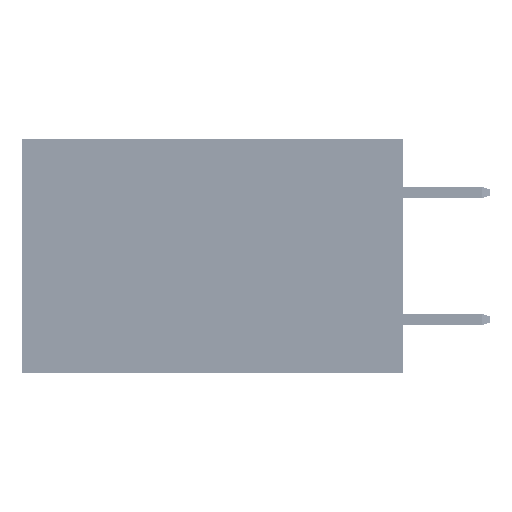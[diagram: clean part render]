
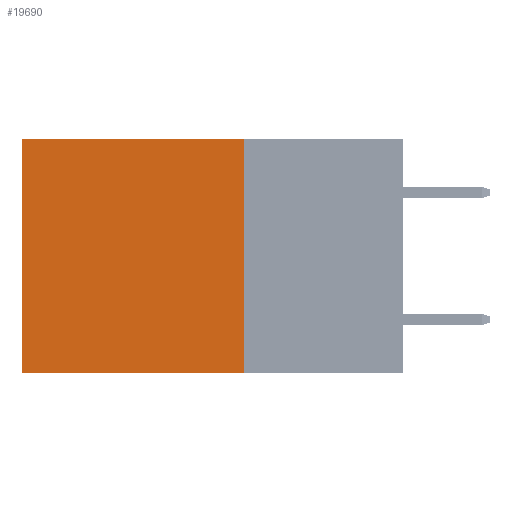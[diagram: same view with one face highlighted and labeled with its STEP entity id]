
A CAD part, left-side view. The second image highlights one B-rep face of the part: STEP entity #19690.
In plain terms, the highlighted planar face has unit normal (-1, 0, 0).
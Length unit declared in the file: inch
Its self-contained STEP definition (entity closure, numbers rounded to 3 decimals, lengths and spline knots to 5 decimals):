
#430 = VECTOR ( 'NONE', #42899, 39.37008 ) ;
#1783 = CARTESIAN_POINT ( 'NONE',  ( 0.2875, 0.6, 0. ) ) ;
#1838 = VECTOR ( 'NONE', #19634, 39.37008 ) ;
#3944 = CARTESIAN_POINT ( 'NONE',  ( 0.2875, 0.25, -0.37 ) ) ;
#4185 = DIRECTION ( 'NONE',  ( 0., 0., -1. ) ) ;
#6712 = DIRECTION ( 'NONE',  ( 0., 0., -1. ) ) ;
#7212 = CARTESIAN_POINT ( 'NONE',  ( 0.2875, 0.25, 0. ) ) ;
#9353 = EDGE_CURVE ( 'NONE', #19038, #37583, #23503, .T. ) ;
#11461 = DIRECTION ( 'NONE',  ( 1., 0., 0. ) ) ;
#12216 = EDGE_CURVE ( 'NONE', #24993, #31007, #19320, .T. ) ;
#14559 = ORIENTED_EDGE ( 'NONE', *, *, #12216, .F. ) ;
#17814 = ORIENTED_EDGE ( 'NONE', *, *, #51083, .F. ) ;
#19038 = VERTEX_POINT ( 'NONE', #46469 ) ;
#19320 = LINE ( 'NONE', #35638, #430 ) ;
#19634 = DIRECTION ( 'NONE',  ( 0., 1., 0. ) ) ;
#19690 = ADVANCED_FACE ( 'NONE', ( #31373 ), #31117, .F. ) ;
#21951 = EDGE_CURVE ( 'NONE', #37583, #31007, #27551, .T. ) ;
#22494 = LINE ( 'NONE', #26634, #33222 ) ;
#23503 = LINE ( 'NONE', #7212, #1838 ) ;
#23660 = DIRECTION ( 'NONE',  ( 0., 0., -1. ) ) ;
#24993 = VERTEX_POINT ( 'NONE', #3944 ) ;
#26634 = CARTESIAN_POINT ( 'NONE',  ( 0.2875, 0.25, 0. ) ) ;
#27551 = LINE ( 'NONE', #51126, #47798 ) ;
#28004 = CARTESIAN_POINT ( 'NONE',  ( 0.2875, 0.25, 0. ) ) ;
#31007 = VERTEX_POINT ( 'NONE', #48733 ) ;
#31117 = PLANE ( 'NONE',  #31920 ) ;
#31373 = FACE_OUTER_BOUND ( 'NONE', #41335, .T. ) ;
#31920 = AXIS2_PLACEMENT_3D ( 'NONE', #28004, #11461, #4185 ) ;
#33222 = VECTOR ( 'NONE', #6712, 39.37008 ) ;
#35638 = CARTESIAN_POINT ( 'NONE',  ( 0.2875, 0.25, -0.37 ) ) ;
#37583 = VERTEX_POINT ( 'NONE', #1783 ) ;
#40509 = ORIENTED_EDGE ( 'NONE', *, *, #9353, .T. ) ;
#41335 = EDGE_LOOP ( 'NONE', ( #41527, #14559, #17814, #40509 ) ) ;
#41527 = ORIENTED_EDGE ( 'NONE', *, *, #21951, .T. ) ;
#42899 = DIRECTION ( 'NONE',  ( 0., 1., 0. ) ) ;
#46469 = CARTESIAN_POINT ( 'NONE',  ( 0.2875, 0.25, 0. ) ) ;
#47798 = VECTOR ( 'NONE', #23660, 39.37008 ) ;
#48733 = CARTESIAN_POINT ( 'NONE',  ( 0.2875, 0.6, -0.37 ) ) ;
#51083 = EDGE_CURVE ( 'NONE', #19038, #24993, #22494, .T. ) ;
#51126 = CARTESIAN_POINT ( 'NONE',  ( 0.2875, 0.6, 0. ) ) ;
